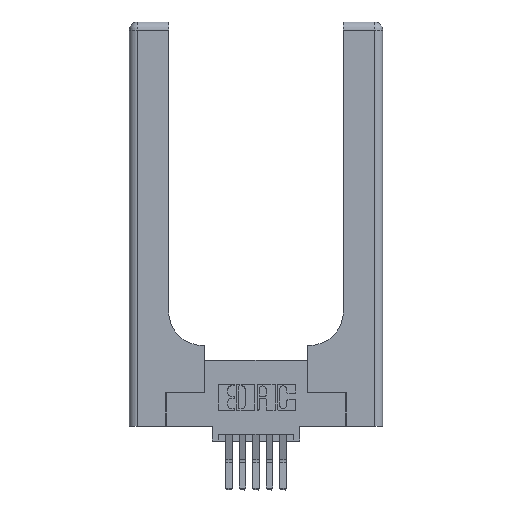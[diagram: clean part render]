
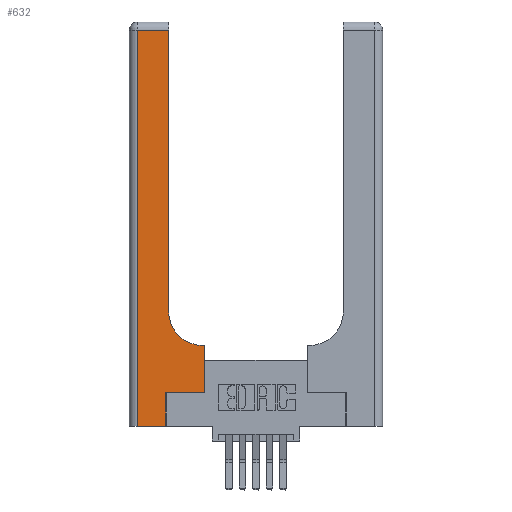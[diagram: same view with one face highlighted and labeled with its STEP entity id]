
A CAD part, top view. The second image highlights one B-rep face of the part: STEP entity #632.
In plain terms, the highlighted planar face has unit normal (0, 0, 1).
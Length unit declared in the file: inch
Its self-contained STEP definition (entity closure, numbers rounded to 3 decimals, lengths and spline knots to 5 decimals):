
#20 = VERTEX_POINT ( 'NONE', #1304 ) ;
#31 = VERTEX_POINT ( 'NONE', #11297 ) ;
#107 = EDGE_CURVE ( 'NONE', #9469, #11381, #14320, .T. ) ;
#452 = DIRECTION ( 'NONE',  ( 1., 0., 0. ) ) ;
#624 = VECTOR ( 'NONE', #7994, 39.37008 ) ;
#632 = ADVANCED_FACE ( 'NONE', ( #11567 ), #1272, .F. ) ;
#1182 = CARTESIAN_POINT ( 'NONE',  ( 0., 3., 0.37 ) ) ;
#1272 = PLANE ( 'NONE',  #6833 ) ;
#1304 = CARTESIAN_POINT ( 'NONE',  ( 0.2915, 0.85, 0.37 ) ) ;
#1556 = CARTESIAN_POINT ( 'NONE',  ( 0.5585, 0.25, 0.37 ) ) ;
#1572 = ORIENTED_EDGE ( 'NONE', *, *, #9863, .T. ) ;
#1629 = VECTOR ( 'NONE', #13792, 39.37008 ) ;
#1657 = DIRECTION ( 'NONE',  ( 0., 1., 0. ) ) ;
#1894 = CARTESIAN_POINT ( 'NONE',  ( 0.06, 3., 0.37 ) ) ;
#2234 = ORIENTED_EDGE ( 'NONE', *, *, #7256, .T. ) ;
#2783 = VECTOR ( 'NONE', #452, 39.37008 ) ;
#2900 = EDGE_CURVE ( 'NONE', #12009, #5954, #5446, .T. ) ;
#3312 = VECTOR ( 'NONE', #7474, 39.37008 ) ;
#3492 = ORIENTED_EDGE ( 'NONE', *, *, #10007, .T. ) ;
#3535 = CARTESIAN_POINT ( 'NONE',  ( 0.269, 0., 0.37 ) ) ;
#3582 = VECTOR ( 'NONE', #3748, 39.37008 ) ;
#3748 = DIRECTION ( 'NONE',  ( 0., 1., 0. ) ) ;
#3995 = EDGE_CURVE ( 'NONE', #11381, #31, #8212, .T. ) ;
#4082 = CARTESIAN_POINT ( 'NONE',  ( 0.269, 0.25, 0.37 ) ) ;
#4421 = ORIENTED_EDGE ( 'NONE', *, *, #10653, .T. ) ;
#4426 = CARTESIAN_POINT ( 'NONE',  ( 0., 0., 0.37 ) ) ;
#4429 = ORIENTED_EDGE ( 'NONE', *, *, #13890, .T. ) ;
#4996 = CARTESIAN_POINT ( 'NONE',  ( 0., 2.94, 0.37 ) ) ;
#5052 = CARTESIAN_POINT ( 'NONE',  ( 0.2915, 0.6, 0.37 ) ) ;
#5093 = AXIS2_PLACEMENT_3D ( 'NONE', #14147, #13104, #6372 ) ;
#5446 = LINE ( 'NONE', #4426, #624 ) ;
#5778 = EDGE_CURVE ( 'NONE', #10271, #12009, #8841, .T. ) ;
#5954 = VERTEX_POINT ( 'NONE', #6344 ) ;
#5975 = LINE ( 'NONE', #9244, #3582 ) ;
#6344 = CARTESIAN_POINT ( 'NONE',  ( 0.269, 0., 0.37 ) ) ;
#6372 = DIRECTION ( 'NONE',  ( 1., 0., 0. ) ) ;
#6709 = DIRECTION ( 'NONE',  ( -1., 0., 0. ) ) ;
#6833 = AXIS2_PLACEMENT_3D ( 'NONE', #1182, #7777, #6709 ) ;
#6953 = CARTESIAN_POINT ( 'NONE',  ( 0.2915, 2.94, 0.37 ) ) ;
#7185 = DIRECTION ( 'NONE',  ( -1., 0., 0. ) ) ;
#7218 = VECTOR ( 'NONE', #7185, 39.37008 ) ;
#7256 = EDGE_CURVE ( 'NONE', #8302, #9469, #7963, .T. ) ;
#7474 = DIRECTION ( 'NONE',  ( 0., -1., 0. ) ) ;
#7734 = CARTESIAN_POINT ( 'NONE',  ( 0.06, 0., 0.37 ) ) ;
#7777 = DIRECTION ( 'NONE',  ( 0., 0., -1. ) ) ;
#7963 = LINE ( 'NONE', #12639, #2783 ) ;
#7985 = CARTESIAN_POINT ( 'NONE',  ( 0.06, 2.94, 0.37 ) ) ;
#7994 = DIRECTION ( 'NONE',  ( 1., 0., 0. ) ) ;
#8071 = LINE ( 'NONE', #3535, #8913 ) ;
#8212 = LINE ( 'NONE', #5052, #1629 ) ;
#8230 = CIRCLE ( 'NONE', #5093, 0.25 ) ;
#8302 = VERTEX_POINT ( 'NONE', #4082 ) ;
#8801 = ORIENTED_EDGE ( 'NONE', *, *, #107, .T. ) ;
#8841 = LINE ( 'NONE', #1894, #3312 ) ;
#8913 = VECTOR ( 'NONE', #11418, 39.37008 ) ;
#9244 = CARTESIAN_POINT ( 'NONE',  ( 0.2915, 3., 0.37 ) ) ;
#9447 = LINE ( 'NONE', #4996, #7218 ) ;
#9469 = VERTEX_POINT ( 'NONE', #11843 ) ;
#9790 = CARTESIAN_POINT ( 'NONE',  ( 0.5585, 0.6, 0.37 ) ) ;
#9863 = EDGE_CURVE ( 'NONE', #20, #12094, #5975, .T. ) ;
#9875 = EDGE_LOOP ( 'NONE', ( #1572, #3492, #12668, #10817, #4429, #2234, #8801, #14222, #4421 ) ) ;
#10007 = EDGE_CURVE ( 'NONE', #12094, #10271, #9447, .T. ) ;
#10271 = VERTEX_POINT ( 'NONE', #7985 ) ;
#10653 = EDGE_CURVE ( 'NONE', #31, #20, #8230, .T. ) ;
#10817 = ORIENTED_EDGE ( 'NONE', *, *, #2900, .T. ) ;
#11071 = VECTOR ( 'NONE', #1657, 39.37008 ) ;
#11297 = CARTESIAN_POINT ( 'NONE',  ( 0.5415, 0.6, 0.37 ) ) ;
#11381 = VERTEX_POINT ( 'NONE', #9790 ) ;
#11418 = DIRECTION ( 'NONE',  ( 0., 1., 0. ) ) ;
#11567 = FACE_OUTER_BOUND ( 'NONE', #9875, .T. ) ;
#11843 = CARTESIAN_POINT ( 'NONE',  ( 0.5585, 0.25, 0.37 ) ) ;
#12009 = VERTEX_POINT ( 'NONE', #7734 ) ;
#12094 = VERTEX_POINT ( 'NONE', #6953 ) ;
#12639 = CARTESIAN_POINT ( 'NONE',  ( 0.269, 0.25, 0.37 ) ) ;
#12668 = ORIENTED_EDGE ( 'NONE', *, *, #5778, .T. ) ;
#13104 = DIRECTION ( 'NONE',  ( 0., 0., -1. ) ) ;
#13792 = DIRECTION ( 'NONE',  ( -1., 0., 0. ) ) ;
#13890 = EDGE_CURVE ( 'NONE', #5954, #8302, #8071, .T. ) ;
#14147 = CARTESIAN_POINT ( 'NONE',  ( 0.5415, 0.85, 0.37 ) ) ;
#14222 = ORIENTED_EDGE ( 'NONE', *, *, #3995, .T. ) ;
#14320 = LINE ( 'NONE', #1556, #11071 ) ;
